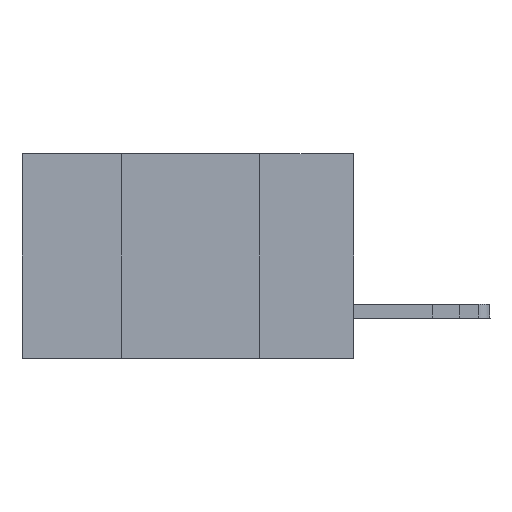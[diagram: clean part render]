
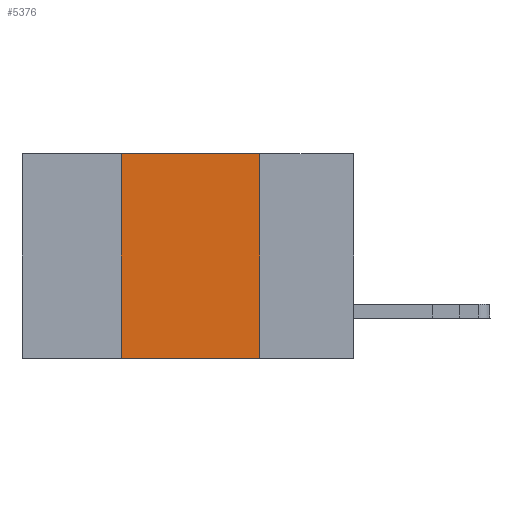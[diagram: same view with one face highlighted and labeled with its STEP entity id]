
A CAD part, left-side view. The second image highlights one B-rep face of the part: STEP entity #5376.
In plain terms, the highlighted planar face has unit normal (-1, 0, 0).
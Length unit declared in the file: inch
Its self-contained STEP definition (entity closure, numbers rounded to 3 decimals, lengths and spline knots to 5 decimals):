
#1039 = ORIENTED_EDGE ( 'NONE', *, *, #22697, .F. ) ;
#1384 = DIRECTION ( 'NONE',  ( 0., 0., 1. ) ) ;
#1783 = EDGE_LOOP ( 'NONE', ( #8925, #21880, #1039, #20627 ) ) ;
#2093 = CARTESIAN_POINT ( 'NONE',  ( 0., 0.17, 0. ) ) ;
#2394 = LINE ( 'NONE', #9525, #19318 ) ;
#3501 = VECTOR ( 'NONE', #1384, 39.37008 ) ;
#4186 = LINE ( 'NONE', #13268, #21189 ) ;
#4748 = VECTOR ( 'NONE', #17588, 39.37008 ) ;
#4990 = EDGE_CURVE ( 'NONE', #7674, #8003, #4186, .T. ) ;
#5376 = ADVANCED_FACE ( 'NONE', ( #18525 ), #17013, .F. ) ;
#6307 = DIRECTION ( 'NONE',  ( 1., 0., 0. ) ) ;
#7674 = VERTEX_POINT ( 'NONE', #2093 ) ;
#8003 = VERTEX_POINT ( 'NONE', #12443 ) ;
#8401 = LINE ( 'NONE', #15830, #3501 ) ;
#8692 = EDGE_CURVE ( 'NONE', #18929, #8003, #10491, .T. ) ;
#8856 = CARTESIAN_POINT ( 'NONE',  ( 0., 0.6, -0.37 ) ) ;
#8925 = ORIENTED_EDGE ( 'NONE', *, *, #4990, .F. ) ;
#9525 = CARTESIAN_POINT ( 'NONE',  ( 0., 0.6, 0. ) ) ;
#9806 = CARTESIAN_POINT ( 'NONE',  ( 0., 0.6, 0. ) ) ;
#10476 = VERTEX_POINT ( 'NONE', #18250 ) ;
#10491 = LINE ( 'NONE', #8856, #4748 ) ;
#10558 = EDGE_CURVE ( 'NONE', #10476, #7674, #2394, .T. ) ;
#12443 = CARTESIAN_POINT ( 'NONE',  ( 0., 0.17, -0.37 ) ) ;
#13160 = DIRECTION ( 'NONE',  ( 0., 0., -1. ) ) ;
#13268 = CARTESIAN_POINT ( 'NONE',  ( 0., 0.17, 0. ) ) ;
#15811 = CARTESIAN_POINT ( 'NONE',  ( 0., 0.42, -0.37 ) ) ;
#15830 = CARTESIAN_POINT ( 'NONE',  ( 0., 0.42, 0. ) ) ;
#16616 = DIRECTION ( 'NONE',  ( 0., -1., 0. ) ) ;
#17013 = PLANE ( 'NONE',  #18977 ) ;
#17131 = DIRECTION ( 'NONE',  ( 0., 0., -1. ) ) ;
#17588 = DIRECTION ( 'NONE',  ( 0., -1., 0. ) ) ;
#18250 = CARTESIAN_POINT ( 'NONE',  ( 0., 0.42, 0. ) ) ;
#18525 = FACE_OUTER_BOUND ( 'NONE', #1783, .T. ) ;
#18929 = VERTEX_POINT ( 'NONE', #15811 ) ;
#18977 = AXIS2_PLACEMENT_3D ( 'NONE', #9806, #6307, #17131 ) ;
#19318 = VECTOR ( 'NONE', #16616, 39.37008 ) ;
#20627 = ORIENTED_EDGE ( 'NONE', *, *, #8692, .T. ) ;
#21189 = VECTOR ( 'NONE', #13160, 39.37008 ) ;
#21880 = ORIENTED_EDGE ( 'NONE', *, *, #10558, .F. ) ;
#22697 = EDGE_CURVE ( 'NONE', #18929, #10476, #8401, .T. ) ;
